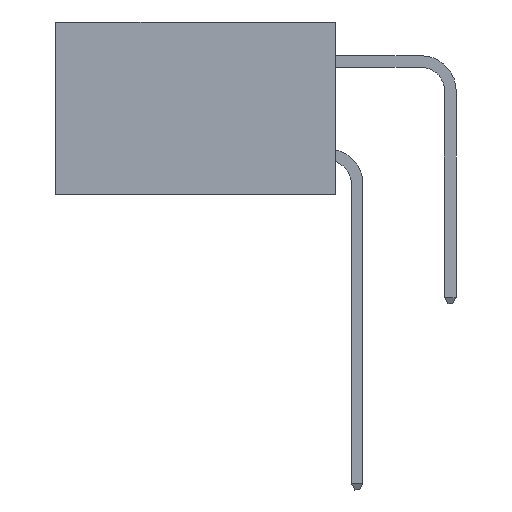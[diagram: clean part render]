
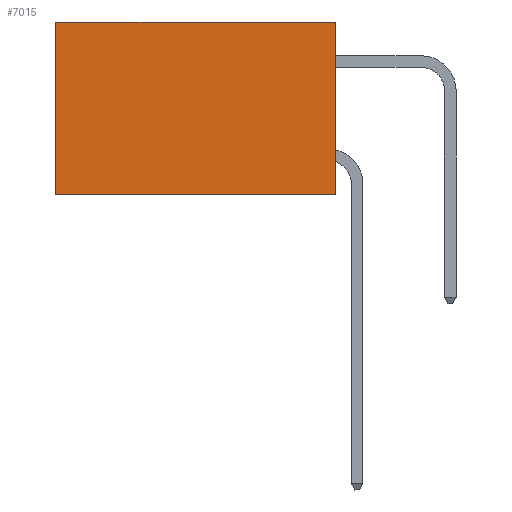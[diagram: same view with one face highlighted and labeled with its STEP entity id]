
A CAD part, left-side view. The second image highlights one B-rep face of the part: STEP entity #7015.
In plain terms, the highlighted planar face has unit normal (-1, 0, 0).
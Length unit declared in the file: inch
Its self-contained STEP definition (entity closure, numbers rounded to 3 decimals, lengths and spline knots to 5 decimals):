
#411 = CARTESIAN_POINT ( 'NONE',  ( 0.2875, 0., 0. ) ) ;
#507 = VECTOR ( 'NONE', #4560, 39.37008 ) ;
#969 = FACE_OUTER_BOUND ( 'NONE', #9577, .T. ) ;
#1184 = CARTESIAN_POINT ( 'NONE',  ( 0.2875, 0.6, 0. ) ) ;
#1188 = ORIENTED_EDGE ( 'NONE', *, *, #3924, .T. ) ;
#1284 = DIRECTION ( 'NONE',  ( 0., 0., -1. ) ) ;
#1820 = CARTESIAN_POINT ( 'NONE',  ( 0.2875, 0.6, -0.37 ) ) ;
#1914 = DIRECTION ( 'NONE',  ( 0., 0., -1. ) ) ;
#1934 = DIRECTION ( 'NONE',  ( 0., 0., -1. ) ) ;
#2425 = CARTESIAN_POINT ( 'NONE',  ( 0.2875, 0., 0. ) ) ;
#2633 = LINE ( 'NONE', #3785, #7350 ) ;
#2858 = EDGE_CURVE ( 'NONE', #11369, #6492, #4075, .T. ) ;
#3785 = CARTESIAN_POINT ( 'NONE',  ( 0.2875, 0.6, 0. ) ) ;
#3886 = AXIS2_PLACEMENT_3D ( 'NONE', #411, #5910, #1914 ) ;
#3924 = EDGE_CURVE ( 'NONE', #11369, #5754, #9985, .T. ) ;
#4075 = LINE ( 'NONE', #2425, #6724 ) ;
#4301 = ORIENTED_EDGE ( 'NONE', *, *, #2858, .F. ) ;
#4560 = DIRECTION ( 'NONE',  ( 0., 1., 0. ) ) ;
#4671 = CARTESIAN_POINT ( 'NONE',  ( 0.2875, 0., -0.37 ) ) ;
#4773 = CARTESIAN_POINT ( 'NONE',  ( 0.2875, 0., 0. ) ) ;
#5680 = DIRECTION ( 'NONE',  ( 0., 1., 0. ) ) ;
#5754 = VERTEX_POINT ( 'NONE', #1184 ) ;
#5910 = DIRECTION ( 'NONE',  ( 1., 0., 0. ) ) ;
#6492 = VERTEX_POINT ( 'NONE', #8613 ) ;
#6724 = VECTOR ( 'NONE', #1284, 39.37008 ) ;
#7015 = ADVANCED_FACE ( 'NONE', ( #969 ), #7517, .F. ) ;
#7023 = CARTESIAN_POINT ( 'NONE',  ( 0.2875, 0., 0. ) ) ;
#7350 = VECTOR ( 'NONE', #1934, 39.37008 ) ;
#7517 = PLANE ( 'NONE',  #3886 ) ;
#8109 = ORIENTED_EDGE ( 'NONE', *, *, #11488, .F. ) ;
#8203 = VERTEX_POINT ( 'NONE', #1820 ) ;
#8613 = CARTESIAN_POINT ( 'NONE',  ( 0.2875, 0., -0.37 ) ) ;
#8858 = ORIENTED_EDGE ( 'NONE', *, *, #9294, .T. ) ;
#9291 = LINE ( 'NONE', #4671, #507 ) ;
#9294 = EDGE_CURVE ( 'NONE', #5754, #8203, #2633, .T. ) ;
#9577 = EDGE_LOOP ( 'NONE', ( #8858, #8109, #4301, #1188 ) ) ;
#9985 = LINE ( 'NONE', #4773, #11236 ) ;
#11236 = VECTOR ( 'NONE', #5680, 39.37008 ) ;
#11369 = VERTEX_POINT ( 'NONE', #7023 ) ;
#11488 = EDGE_CURVE ( 'NONE', #6492, #8203, #9291, .T. ) ;
